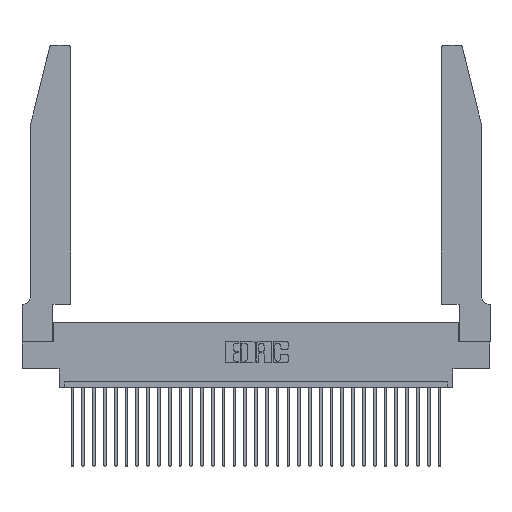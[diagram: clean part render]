
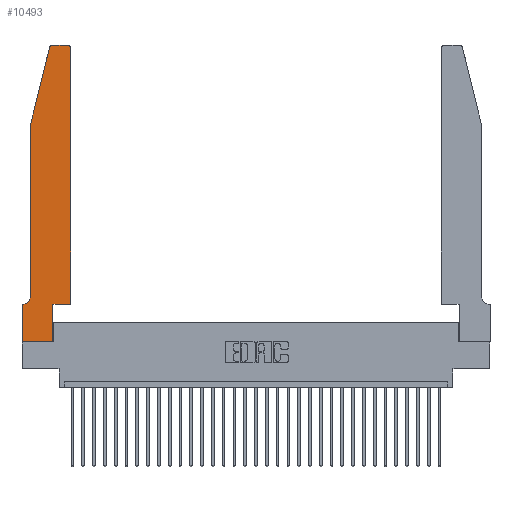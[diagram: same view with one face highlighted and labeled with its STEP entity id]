
A CAD part, top view. The second image highlights one B-rep face of the part: STEP entity #10493.
In plain terms, the highlighted planar face has unit normal (0, 0, 1).
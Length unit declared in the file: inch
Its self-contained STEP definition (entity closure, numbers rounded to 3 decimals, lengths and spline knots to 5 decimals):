
#469 = LINE ( 'NONE', #9720, #12182 ) ;
#526 = DIRECTION ( 'NONE',  ( -0.239, -0.971, 0. ) ) ;
#675 = FACE_OUTER_BOUND ( 'NONE', #6909, .T. ) ;
#793 = DIRECTION ( 'NONE',  ( 0., 0., 1. ) ) ;
#1502 = VECTOR ( 'NONE', #19698, 39.37008 ) ;
#1937 = ORIENTED_EDGE ( 'NONE', *, *, #10319, .T. ) ;
#2245 = LINE ( 'NONE', #6613, #27166 ) ;
#2576 = LINE ( 'NONE', #14247, #23978 ) ;
#3495 = VERTEX_POINT ( 'NONE', #9461 ) ;
#3859 = VERTEX_POINT ( 'NONE', #24630 ) ;
#3924 = ORIENTED_EDGE ( 'NONE', *, *, #5970, .T. ) ;
#4345 = DIRECTION ( 'NONE',  ( 0., -1., 0. ) ) ;
#4535 = EDGE_CURVE ( 'NONE', #3495, #21685, #12647, .T. ) ;
#4646 = CARTESIAN_POINT ( 'NONE',  ( 0.2605, 2.75, 0.37 ) ) ;
#4722 = CARTESIAN_POINT ( 'NONE',  ( 0.2865, 0.35, 0.37 ) ) ;
#4873 = ORIENTED_EDGE ( 'NONE', *, *, #4535, .T. ) ;
#5579 = EDGE_CURVE ( 'NONE', #21685, #27110, #469, .T. ) ;
#5859 = AXIS2_PLACEMENT_3D ( 'NONE', #23738, #13422, #11044 ) ;
#5939 = LINE ( 'NONE', #19026, #31248 ) ;
#5970 = EDGE_CURVE ( 'NONE', #3859, #8609, #29622, .T. ) ;
#6240 = CARTESIAN_POINT ( 'NONE',  ( 0.2865, 0.35, 0.37 ) ) ;
#6489 = CARTESIAN_POINT ( 'NONE',  ( 0., 0., 0.37 ) ) ;
#6613 = CARTESIAN_POINT ( 'NONE',  ( 0.0755, 2., 0.37 ) ) ;
#6813 = VECTOR ( 'NONE', #526, 39.37008 ) ;
#6909 = EDGE_LOOP ( 'NONE', ( #3924, #29966, #8641, #1937, #18064, #10997, #29182, #19522, #4873, #25650, #8179, #15437 ) ) ;
#8076 = CIRCLE ( 'NONE', #22576, 0.03 ) ;
#8121 = VERTEX_POINT ( 'NONE', #6489 ) ;
#8179 = ORIENTED_EDGE ( 'NONE', *, *, #13365, .T. ) ;
#8526 = EDGE_CURVE ( 'NONE', #30585, #13838, #14872, .T. ) ;
#8609 = VERTEX_POINT ( 'NONE', #30899 ) ;
#8641 = ORIENTED_EDGE ( 'NONE', *, *, #32020, .T. ) ;
#8763 = CARTESIAN_POINT ( 'NONE',  ( 0., 0., 0.37 ) ) ;
#8926 = DIRECTION ( 'NONE',  ( 1., 0., 0. ) ) ;
#9223 = EDGE_CURVE ( 'NONE', #24592, #3859, #20199, .T. ) ;
#9373 = LINE ( 'NONE', #8763, #23353 ) ;
#9461 = CARTESIAN_POINT ( 'NONE',  ( 0.2865, 0., 0.37 ) ) ;
#9720 = CARTESIAN_POINT ( 'NONE',  ( 0.4505, 0.35, 0.37 ) ) ;
#9948 = EDGE_CURVE ( 'NONE', #13838, #18600, #31052, .T. ) ;
#10210 = DIRECTION ( 'NONE',  ( 0., 0., -1. ) ) ;
#10319 = EDGE_CURVE ( 'NONE', #26639, #30585, #2245, .T. ) ;
#10493 = ADVANCED_FACE ( 'NONE', ( #675 ), #28192, .T. ) ;
#10511 = EDGE_CURVE ( 'NONE', #8609, #24813, #8076, .T. ) ;
#10997 = ORIENTED_EDGE ( 'NONE', *, *, #9948, .T. ) ;
#11044 = DIRECTION ( 'NONE',  ( 1., 0., 0. ) ) ;
#11340 = AXIS2_PLACEMENT_3D ( 'NONE', #13411, #28300, #25352 ) ;
#11765 = CARTESIAN_POINT ( 'NONE',  ( 0.4505, 2.72, 0.37 ) ) ;
#12182 = VECTOR ( 'NONE', #19694, 39.37008 ) ;
#12647 = LINE ( 'NONE', #4722, #14566 ) ;
#13365 = EDGE_CURVE ( 'NONE', #27110, #24592, #5939, .T. ) ;
#13411 = CARTESIAN_POINT ( 'NONE',  ( 0., 0.35, 0.37 ) ) ;
#13422 = DIRECTION ( 'NONE',  ( 0., 0., 1. ) ) ;
#13838 = VERTEX_POINT ( 'NONE', #25836 ) ;
#14247 = CARTESIAN_POINT ( 'NONE',  ( 0., 0., 0.37 ) ) ;
#14566 = VECTOR ( 'NONE', #27133, 39.37008 ) ;
#14872 = CIRCLE ( 'NONE', #30636, 0.07 ) ;
#15437 = ORIENTED_EDGE ( 'NONE', *, *, #9223, .T. ) ;
#16403 = VECTOR ( 'NONE', #26715, 39.37008 ) ;
#16671 = DIRECTION ( 'NONE',  ( 0., 1., 0. ) ) ;
#17586 = EDGE_CURVE ( 'NONE', #18600, #8121, #9373, .T. ) ;
#18064 = ORIENTED_EDGE ( 'NONE', *, *, #8526, .T. ) ;
#18103 = CARTESIAN_POINT ( 'NONE',  ( 0.284, 2.72, 0.37 ) ) ;
#18600 = VERTEX_POINT ( 'NONE', #23877 ) ;
#19026 = CARTESIAN_POINT ( 'NONE',  ( 0.4505, 0.35, 0.37 ) ) ;
#19522 = ORIENTED_EDGE ( 'NONE', *, *, #19977, .T. ) ;
#19694 = DIRECTION ( 'NONE',  ( 1., 0., 0. ) ) ;
#19698 = DIRECTION ( 'NONE',  ( -1., 0., 0. ) ) ;
#19977 = EDGE_CURVE ( 'NONE', #8121, #3495, #2576, .T. ) ;
#20037 = LINE ( 'NONE', #26969, #6813 ) ;
#20199 = CIRCLE ( 'NONE', #5859, 0.03 ) ;
#20727 = CARTESIAN_POINT ( 'NONE',  ( 0.25487, 2.72718, 0.37 ) ) ;
#21685 = VERTEX_POINT ( 'NONE', #6240 ) ;
#22576 = AXIS2_PLACEMENT_3D ( 'NONE', #18103, #793, #30369 ) ;
#22611 = CARTESIAN_POINT ( 'NONE',  ( 0.0755, 0.42, 0.37 ) ) ;
#23353 = VECTOR ( 'NONE', #28335, 39.37008 ) ;
#23738 = CARTESIAN_POINT ( 'NONE',  ( 0.4205, 2.72, 0.37 ) ) ;
#23877 = CARTESIAN_POINT ( 'NONE',  ( 0., 0.35, 0.37 ) ) ;
#23978 = VECTOR ( 'NONE', #8926, 39.37008 ) ;
#24592 = VERTEX_POINT ( 'NONE', #11765 ) ;
#24630 = CARTESIAN_POINT ( 'NONE',  ( 0.4205, 2.75, 0.37 ) ) ;
#24813 = VERTEX_POINT ( 'NONE', #20727 ) ;
#25155 = CARTESIAN_POINT ( 'NONE',  ( 0.0055, 0.42, 0.37 ) ) ;
#25352 = DIRECTION ( 'NONE',  ( 1., 0., 0. ) ) ;
#25650 = ORIENTED_EDGE ( 'NONE', *, *, #5579, .T. ) ;
#25836 = CARTESIAN_POINT ( 'NONE',  ( 0.0055, 0.35, 0.37 ) ) ;
#26639 = VERTEX_POINT ( 'NONE', #27905 ) ;
#26715 = DIRECTION ( 'NONE',  ( -1., 0., 0. ) ) ;
#26969 = CARTESIAN_POINT ( 'NONE',  ( 0.0755, 2., 0.37 ) ) ;
#27110 = VERTEX_POINT ( 'NONE', #27467 ) ;
#27133 = DIRECTION ( 'NONE',  ( 0., 1., 0. ) ) ;
#27166 = VECTOR ( 'NONE', #4345, 39.37008 ) ;
#27467 = CARTESIAN_POINT ( 'NONE',  ( 0.4505, 0.35, 0.37 ) ) ;
#27572 = DIRECTION ( 'NONE',  ( -1., 0., 0. ) ) ;
#27905 = CARTESIAN_POINT ( 'NONE',  ( 0.0755, 2., 0.37 ) ) ;
#28192 = PLANE ( 'NONE',  #11340 ) ;
#28300 = DIRECTION ( 'NONE',  ( 0., 0., 1. ) ) ;
#28335 = DIRECTION ( 'NONE',  ( 0., -1., 0. ) ) ;
#29182 = ORIENTED_EDGE ( 'NONE', *, *, #17586, .T. ) ;
#29622 = LINE ( 'NONE', #4646, #16403 ) ;
#29966 = ORIENTED_EDGE ( 'NONE', *, *, #10511, .T. ) ;
#30369 = DIRECTION ( 'NONE',  ( 1., 0., 0. ) ) ;
#30585 = VERTEX_POINT ( 'NONE', #22611 ) ;
#30636 = AXIS2_PLACEMENT_3D ( 'NONE', #25155, #10210, #27572 ) ;
#30899 = CARTESIAN_POINT ( 'NONE',  ( 0.284, 2.75, 0.37 ) ) ;
#31052 = LINE ( 'NONE', #31199, #1502 ) ;
#31199 = CARTESIAN_POINT ( 'NONE',  ( 0.0755, 0.35, 0.37 ) ) ;
#31248 = VECTOR ( 'NONE', #16671, 39.37008 ) ;
#32020 = EDGE_CURVE ( 'NONE', #24813, #26639, #20037, .T. ) ;
